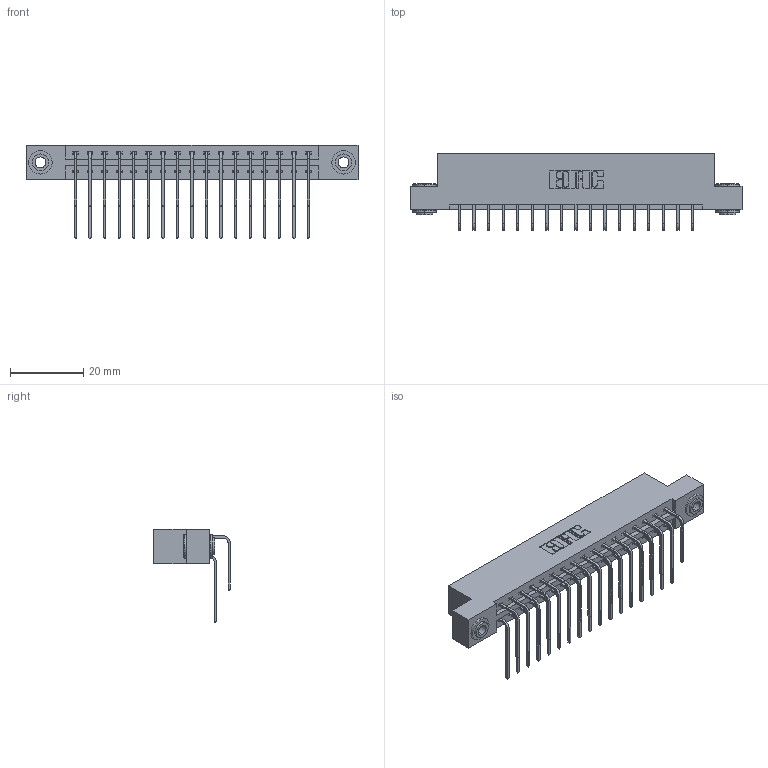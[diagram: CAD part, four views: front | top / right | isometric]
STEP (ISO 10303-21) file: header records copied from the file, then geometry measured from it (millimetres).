
FILE_DESCRIPTION (( 'STEP AP203' ), '1' );
FILE_NAME ('337-034-559-203.STEP', '2018-08-07T19:24:34', ( '' ), ( '' ), 'SwSTEP 2.0', 'SolidWorks 2016', '' );
FILE_SCHEMA (( 'CONFIG_CONTROL_DESIGN' ));
Length unit declared in the file: inch
Products named in the file (5): 337-034-559-203; 337 Part_Flush Mounting Lugs - 0.156 Dia-TH; 345-292-001_558 559 Tail - 1; 345-292-001_559 Tail - 2; 345-250-002_345-250-002-102
Assembly tree (37 placements, depth 2):
  337-034-559-203
    337 Part_Flush Mounting Lugs - 0.156 Dia-TH
    345-292-001_558 559 Tail - 1  x17
    345-292-001_559 Tail - 2  x17
    345-250-002_345-250-002-102  x2
Bounding box: 90.37 x 20.9 x 25.53 mm (x, y, z)
Volume: 9407 mm3; surface area: 11601 mm2
Topology: 37 solids, 37 shells, 2056 faces, 6065 edges, 3994 vertices
Faces by surface type: plane 1440, cylinder 608, cone 8
Entity records: 18848 total; most frequent: CARTESIAN_POINT 3216, ORIENTED_EDGE 3094, DIRECTION 2797, EDGE_CURVE 1547, VECTOR 1355, LINE 1355, VERTEX_POINT 1026, AXIS2_PLACEMENT_3D 721
